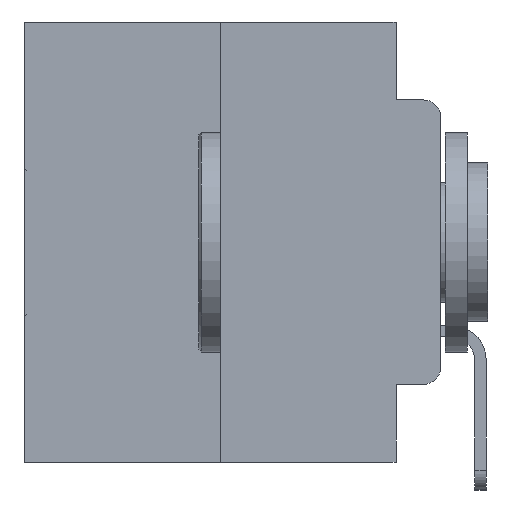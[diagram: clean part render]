
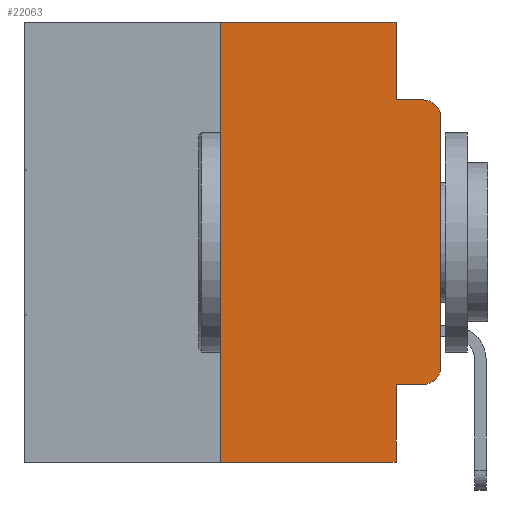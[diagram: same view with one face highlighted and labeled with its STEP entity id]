
A CAD part, left-side view. The second image highlights one B-rep face of the part: STEP entity #22063.
In plain terms, the highlighted planar face has unit normal (-1, 0, 0).
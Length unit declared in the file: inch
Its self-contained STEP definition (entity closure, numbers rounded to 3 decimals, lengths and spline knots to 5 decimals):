
#580 = EDGE_CURVE ( 'NONE', #2035, #4633, #6653, .T. ) ;
#671 = EDGE_CURVE ( 'NONE', #8848, #4354, #10962, .T. ) ;
#764 = CARTESIAN_POINT ( 'NONE',  ( 0., 0.473, -0.5 ) ) ;
#1382 = CARTESIAN_POINT ( 'NONE',  ( 0., 0., -0.1085 ) ) ;
#1604 = ORIENTED_EDGE ( 'NONE', *, *, #580, .T. ) ;
#2035 = VERTEX_POINT ( 'NONE', #16222 ) ;
#2279 = CARTESIAN_POINT ( 'NONE',  ( 0., 0.051, -0.0885 ) ) ;
#2560 = FACE_OUTER_BOUND ( 'NONE', #16903, .T. ) ;
#3194 = LINE ( 'NONE', #17034, #11142 ) ;
#3653 = CARTESIAN_POINT ( 'NONE',  ( 0., 0.02, -0.0885 ) ) ;
#4137 = LINE ( 'NONE', #764, #11676 ) ;
#4354 = VERTEX_POINT ( 'NONE', #24582 ) ;
#4633 = VERTEX_POINT ( 'NONE', #28188 ) ;
#5785 = CARTESIAN_POINT ( 'NONE',  ( 0., 0.051, 0. ) ) ;
#5888 = CARTESIAN_POINT ( 'NONE',  ( 0., 0.02, -0.1085 ) ) ;
#6055 = DIRECTION ( 'NONE',  ( 0., 0., -1. ) ) ;
#6164 = DIRECTION ( 'NONE',  ( 1., 0., 0. ) ) ;
#6332 = VECTOR ( 'NONE', #15533, 39.37008 ) ;
#6554 = AXIS2_PLACEMENT_3D ( 'NONE', #5888, #12808, #12918 ) ;
#6653 = CIRCLE ( 'NONE', #18325, 0.02 ) ;
#7082 = ORIENTED_EDGE ( 'NONE', *, *, #20941, .F. ) ;
#7538 = VERTEX_POINT ( 'NONE', #1382 ) ;
#7554 = VERTEX_POINT ( 'NONE', #26950 ) ;
#7728 = DIRECTION ( 'NONE',  ( 0., -1., 0. ) ) ;
#8092 = CARTESIAN_POINT ( 'NONE',  ( 0., 0.051, -0.0885 ) ) ;
#8352 = PLANE ( 'NONE',  #14468 ) ;
#8472 = DIRECTION ( 'NONE',  ( -1., 0., 0. ) ) ;
#8848 = VERTEX_POINT ( 'NONE', #25919 ) ;
#8991 = EDGE_CURVE ( 'NONE', #24750, #2035, #3194, .T. ) ;
#9904 = ORIENTED_EDGE ( 'NONE', *, *, #671, .F. ) ;
#10407 = DIRECTION ( 'NONE',  ( 0., 0., -1. ) ) ;
#10687 = CARTESIAN_POINT ( 'NONE',  ( 0., 0.02, -0.3915 ) ) ;
#10839 = DIRECTION ( 'NONE',  ( 0., 0., 1. ) ) ;
#10962 = LINE ( 'NONE', #25888, #26766 ) ;
#11089 = CARTESIAN_POINT ( 'NONE',  ( 0., 0.473, 0. ) ) ;
#11142 = VECTOR ( 'NONE', #21743, 39.37008 ) ;
#11454 = EDGE_CURVE ( 'NONE', #4354, #21251, #18120, .T. ) ;
#11676 = VECTOR ( 'NONE', #7728, 39.37008 ) ;
#12746 = ORIENTED_EDGE ( 'NONE', *, *, #15611, .T. ) ;
#12808 = DIRECTION ( 'NONE',  ( -1., 0., 0. ) ) ;
#12918 = DIRECTION ( 'NONE',  ( 0., 0., -1. ) ) ;
#12994 = DIRECTION ( 'NONE',  ( 0., 0., -1. ) ) ;
#13091 = CIRCLE ( 'NONE', #6554, 0.02 ) ;
#13229 = CARTESIAN_POINT ( 'NONE',  ( 0., 0., 0. ) ) ;
#13287 = CARTESIAN_POINT ( 'NONE',  ( 0., 0.051, 0. ) ) ;
#13895 = LINE ( 'NONE', #14851, #21759 ) ;
#14025 = DIRECTION ( 'NONE',  ( 0., -1., 0. ) ) ;
#14468 = AXIS2_PLACEMENT_3D ( 'NONE', #24505, #6164, #6055 ) ;
#14851 = CARTESIAN_POINT ( 'NONE',  ( 0., 0.051, 0. ) ) ;
#15235 = DIRECTION ( 'NONE',  ( 0., 0., -1. ) ) ;
#15302 = EDGE_CURVE ( 'NONE', #7538, #26009, #13091, .T. ) ;
#15533 = DIRECTION ( 'NONE',  ( 0., -1., 0. ) ) ;
#15611 = EDGE_CURVE ( 'NONE', #8848, #7554, #4137, .T. ) ;
#16222 = CARTESIAN_POINT ( 'NONE',  ( 0., 0.02, -0.4115 ) ) ;
#16582 = ORIENTED_EDGE ( 'NONE', *, *, #8991, .T. ) ;
#16903 = EDGE_LOOP ( 'NONE', ( #22484, #27407, #7082, #25794, #23021, #9904, #12746, #18179, #16582, #1604 ) ) ;
#17034 = CARTESIAN_POINT ( 'NONE',  ( 0., 0.051, -0.4115 ) ) ;
#18120 = LINE ( 'NONE', #11089, #6332 ) ;
#18179 = ORIENTED_EDGE ( 'NONE', *, *, #26067, .F. ) ;
#18325 = AXIS2_PLACEMENT_3D ( 'NONE', #10687, #8472, #15235 ) ;
#18419 = VERTEX_POINT ( 'NONE', #8092 ) ;
#20246 = LINE ( 'NONE', #2279, #28942 ) ;
#20941 = EDGE_CURVE ( 'NONE', #18419, #26009, #20246, .T. ) ;
#21251 = VERTEX_POINT ( 'NONE', #5785 ) ;
#21743 = DIRECTION ( 'NONE',  ( 0., -1., 0. ) ) ;
#21759 = VECTOR ( 'NONE', #10407, 39.37008 ) ;
#22063 = ADVANCED_FACE ( 'NONE', ( #2560 ), #8352, .F. ) ;
#22184 = LINE ( 'NONE', #13287, #29835 ) ;
#22484 = ORIENTED_EDGE ( 'NONE', *, *, #29278, .T. ) ;
#23021 = ORIENTED_EDGE ( 'NONE', *, *, #11454, .F. ) ;
#24505 = CARTESIAN_POINT ( 'NONE',  ( 0., 0.473, 0. ) ) ;
#24582 = CARTESIAN_POINT ( 'NONE',  ( 0., 0.25, 0. ) ) ;
#24641 = EDGE_CURVE ( 'NONE', #21251, #18419, #13895, .T. ) ;
#24750 = VERTEX_POINT ( 'NONE', #29028 ) ;
#24800 = LINE ( 'NONE', #13229, #27002 ) ;
#25508 = DIRECTION ( 'NONE',  ( 0., 0., 1. ) ) ;
#25794 = ORIENTED_EDGE ( 'NONE', *, *, #24641, .F. ) ;
#25888 = CARTESIAN_POINT ( 'NONE',  ( 0., 0.25, 0. ) ) ;
#25919 = CARTESIAN_POINT ( 'NONE',  ( 0., 0.25, -0.5 ) ) ;
#26009 = VERTEX_POINT ( 'NONE', #3653 ) ;
#26067 = EDGE_CURVE ( 'NONE', #24750, #7554, #22184, .T. ) ;
#26766 = VECTOR ( 'NONE', #25508, 39.37008 ) ;
#26950 = CARTESIAN_POINT ( 'NONE',  ( 0., 0.051, -0.5 ) ) ;
#27002 = VECTOR ( 'NONE', #10839, 39.37008 ) ;
#27407 = ORIENTED_EDGE ( 'NONE', *, *, #15302, .T. ) ;
#28188 = CARTESIAN_POINT ( 'NONE',  ( 0., 0., -0.3915 ) ) ;
#28942 = VECTOR ( 'NONE', #14025, 39.37008 ) ;
#29028 = CARTESIAN_POINT ( 'NONE',  ( 0., 0.051, -0.4115 ) ) ;
#29278 = EDGE_CURVE ( 'NONE', #4633, #7538, #24800, .T. ) ;
#29835 = VECTOR ( 'NONE', #12994, 39.37008 ) ;
